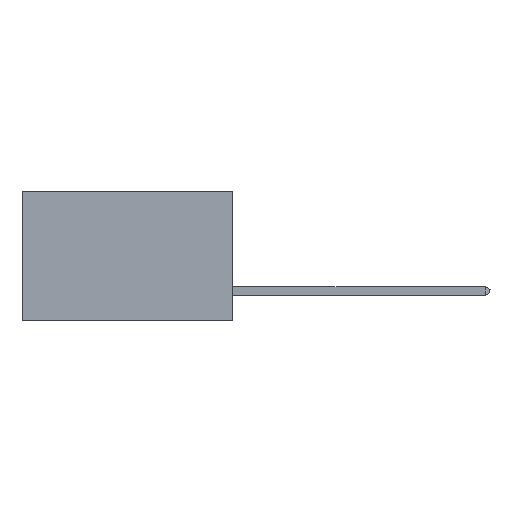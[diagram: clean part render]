
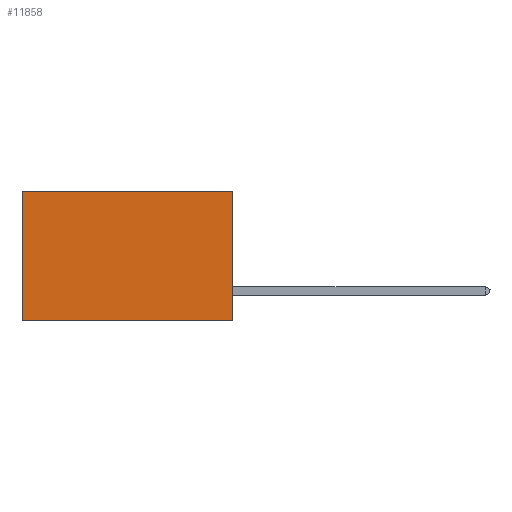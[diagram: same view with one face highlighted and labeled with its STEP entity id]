
A CAD part, left-side view. The second image highlights one B-rep face of the part: STEP entity #11858.
In plain terms, the highlighted planar face has unit normal (-1, 0, 0).
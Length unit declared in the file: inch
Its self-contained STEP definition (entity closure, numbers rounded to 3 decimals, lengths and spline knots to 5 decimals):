
#625 = LINE ( 'NONE', #22562, #11162 ) ;
#667 = VERTEX_POINT ( 'NONE', #7444 ) ;
#3032 = ORIENTED_EDGE ( 'NONE', *, *, #10286, .T. ) ;
#3258 = CARTESIAN_POINT ( 'NONE',  ( 0.2875, 0.6, 0. ) ) ;
#3904 = CARTESIAN_POINT ( 'NONE',  ( 0.2875, 0.6, -0.37 ) ) ;
#4740 = LINE ( 'NONE', #15876, #23745 ) ;
#4990 = EDGE_CURVE ( 'NONE', #6850, #667, #4740, .T. ) ;
#5288 = DIRECTION ( 'NONE',  ( 0., 1., 0. ) ) ;
#6062 = FACE_OUTER_BOUND ( 'NONE', #19395, .T. ) ;
#6322 = EDGE_CURVE ( 'NONE', #20908, #26283, #21623, .T. ) ;
#6850 = VERTEX_POINT ( 'NONE', #16163 ) ;
#7444 = CARTESIAN_POINT ( 'NONE',  ( 0.2875, 0., -0.37 ) ) ;
#8307 = DIRECTION ( 'NONE',  ( 1., 0., 0. ) ) ;
#8883 = VECTOR ( 'NONE', #16906, 39.37008 ) ;
#9278 = AXIS2_PLACEMENT_3D ( 'NONE', #10354, #8307, #25276 ) ;
#10286 = EDGE_CURVE ( 'NONE', #6850, #20908, #25781, .T. ) ;
#10354 = CARTESIAN_POINT ( 'NONE',  ( 0.2875, 0., 0. ) ) ;
#11162 = VECTOR ( 'NONE', #5288, 39.37008 ) ;
#11786 = EDGE_CURVE ( 'NONE', #667, #26283, #625, .T. ) ;
#11858 = ADVANCED_FACE ( 'NONE', ( #6062 ), #14605, .F. ) ;
#14605 = PLANE ( 'NONE',  #9278 ) ;
#15876 = CARTESIAN_POINT ( 'NONE',  ( 0.2875, 0., 0. ) ) ;
#15892 = VECTOR ( 'NONE', #20860, 39.37008 ) ;
#16163 = CARTESIAN_POINT ( 'NONE',  ( 0.2875, 0., 0. ) ) ;
#16906 = DIRECTION ( 'NONE',  ( 0., 1., 0. ) ) ;
#18699 = CARTESIAN_POINT ( 'NONE',  ( 0.2875, 0.6, 0. ) ) ;
#19395 = EDGE_LOOP ( 'NONE', ( #26972, #23420, #27792, #3032 ) ) ;
#20557 = CARTESIAN_POINT ( 'NONE',  ( 0.2875, 0., 0. ) ) ;
#20860 = DIRECTION ( 'NONE',  ( 0., 0., -1. ) ) ;
#20908 = VERTEX_POINT ( 'NONE', #3258 ) ;
#21623 = LINE ( 'NONE', #18699, #15892 ) ;
#22562 = CARTESIAN_POINT ( 'NONE',  ( 0.2875, 0., -0.37 ) ) ;
#22916 = DIRECTION ( 'NONE',  ( 0., 0., -1. ) ) ;
#23420 = ORIENTED_EDGE ( 'NONE', *, *, #11786, .F. ) ;
#23745 = VECTOR ( 'NONE', #22916, 39.37008 ) ;
#25276 = DIRECTION ( 'NONE',  ( 0., 0., -1. ) ) ;
#25781 = LINE ( 'NONE', #20557, #8883 ) ;
#26283 = VERTEX_POINT ( 'NONE', #3904 ) ;
#26972 = ORIENTED_EDGE ( 'NONE', *, *, #6322, .T. ) ;
#27792 = ORIENTED_EDGE ( 'NONE', *, *, #4990, .F. ) ;
